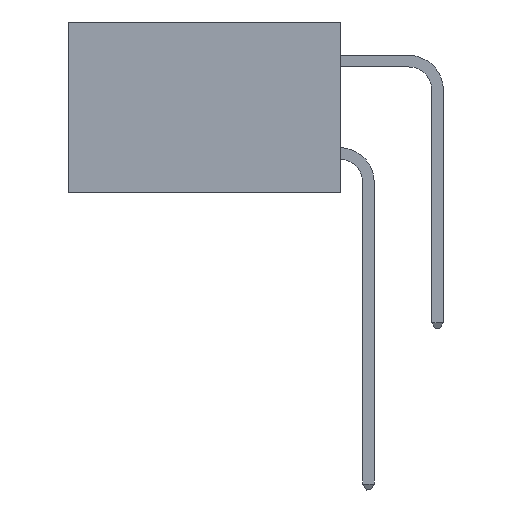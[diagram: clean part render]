
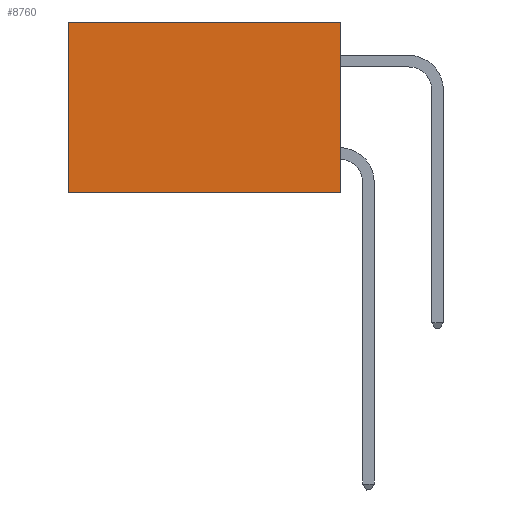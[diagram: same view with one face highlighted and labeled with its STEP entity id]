
A CAD part, left-side view. The second image highlights one B-rep face of the part: STEP entity #8760.
In plain terms, the highlighted planar face has unit normal (-1, 0, 0).
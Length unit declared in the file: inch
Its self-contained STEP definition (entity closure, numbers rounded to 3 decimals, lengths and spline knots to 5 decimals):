
#2508 = VERTEX_POINT ( 'NONE', #14518 ) ;
#2641 = CARTESIAN_POINT ( 'NONE',  ( 0.277, 0.59, 0. ) ) ;
#2897 = VECTOR ( 'NONE', #7092, 39.37008 ) ;
#4045 = EDGE_CURVE ( 'NONE', #2508, #24139, #10720, .T. ) ;
#7092 = DIRECTION ( 'NONE',  ( 0., 1., 0. ) ) ;
#8760 = ADVANCED_FACE ( 'NONE', ( #31767 ), #10487, .F. ) ;
#8776 = CARTESIAN_POINT ( 'NONE',  ( 0.277, 0., -0.37 ) ) ;
#10411 = DIRECTION ( 'NONE',  ( 0., 0., -1. ) ) ;
#10482 = DIRECTION ( 'NONE',  ( 1., 0., 0. ) ) ;
#10487 = PLANE ( 'NONE',  #30474 ) ;
#10720 = LINE ( 'NONE', #8776, #2897 ) ;
#11433 = CARTESIAN_POINT ( 'NONE',  ( 0.277, 0., -0.37 ) ) ;
#12065 = ORIENTED_EDGE ( 'NONE', *, *, #18865, .T. ) ;
#12250 = ORIENTED_EDGE ( 'NONE', *, *, #26304, .T. ) ;
#14001 = VECTOR ( 'NONE', #18458, 39.37008 ) ;
#14205 = CARTESIAN_POINT ( 'NONE',  ( 0.277, 0., 0. ) ) ;
#14518 = CARTESIAN_POINT ( 'NONE',  ( 0.277, 0., -0.37 ) ) ;
#15123 = LINE ( 'NONE', #15796, #14001 ) ;
#15796 = CARTESIAN_POINT ( 'NONE',  ( 0.277, 0., -0.37 ) ) ;
#16339 = CARTESIAN_POINT ( 'NONE',  ( 0.277, 0.59, -0.37 ) ) ;
#16894 = DIRECTION ( 'NONE',  ( 0., 1., 0. ) ) ;
#18347 = CARTESIAN_POINT ( 'NONE',  ( 0.277, 0., 0. ) ) ;
#18458 = DIRECTION ( 'NONE',  ( 0., 0., -1. ) ) ;
#18865 = EDGE_CURVE ( 'NONE', #27306, #24139, #29942, .T. ) ;
#19281 = LINE ( 'NONE', #14205, #32386 ) ;
#19907 = EDGE_LOOP ( 'NONE', ( #12065, #24457, #21999, #12250 ) ) ;
#21289 = VECTOR ( 'NONE', #32067, 39.37008 ) ;
#21999 = ORIENTED_EDGE ( 'NONE', *, *, #31339, .F. ) ;
#24139 = VERTEX_POINT ( 'NONE', #30614 ) ;
#24457 = ORIENTED_EDGE ( 'NONE', *, *, #4045, .F. ) ;
#26304 = EDGE_CURVE ( 'NONE', #33234, #27306, #19281, .T. ) ;
#27306 = VERTEX_POINT ( 'NONE', #2641 ) ;
#29942 = LINE ( 'NONE', #16339, #21289 ) ;
#30474 = AXIS2_PLACEMENT_3D ( 'NONE', #11433, #10482, #10411 ) ;
#30614 = CARTESIAN_POINT ( 'NONE',  ( 0.277, 0.59, -0.37 ) ) ;
#31339 = EDGE_CURVE ( 'NONE', #33234, #2508, #15123, .T. ) ;
#31767 = FACE_OUTER_BOUND ( 'NONE', #19907, .T. ) ;
#32067 = DIRECTION ( 'NONE',  ( 0., 0., -1. ) ) ;
#32386 = VECTOR ( 'NONE', #16894, 39.37008 ) ;
#33234 = VERTEX_POINT ( 'NONE', #18347 ) ;
